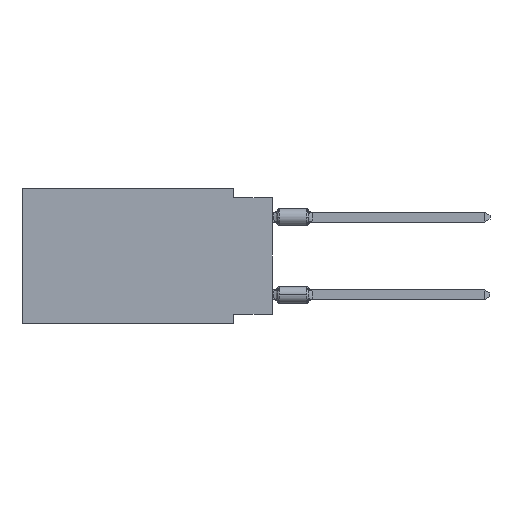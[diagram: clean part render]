
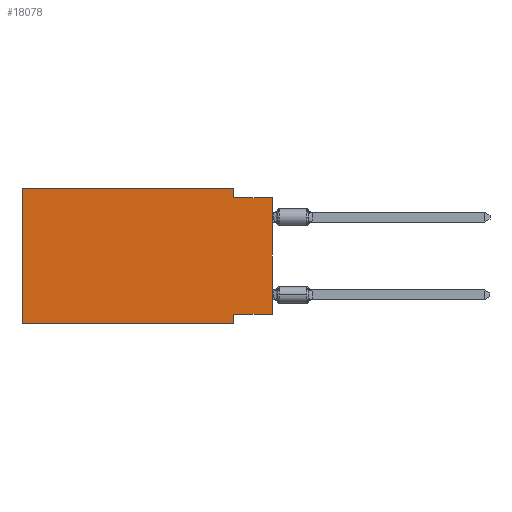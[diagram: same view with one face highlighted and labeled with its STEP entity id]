
A CAD part, left-side view. The second image highlights one B-rep face of the part: STEP entity #18078.
In plain terms, the highlighted planar face has unit normal (-1, 0, 0).
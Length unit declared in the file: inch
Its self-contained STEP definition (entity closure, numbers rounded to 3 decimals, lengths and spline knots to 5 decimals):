
#217 = VECTOR ( 'NONE', #5958, 39.37008 ) ;
#378 = EDGE_CURVE ( 'NONE', #1676, #13019, #11551, .T. ) ;
#433 = ORIENTED_EDGE ( 'NONE', *, *, #378, .F. ) ;
#554 = VERTEX_POINT ( 'NONE', #3143 ) ;
#1120 = CARTESIAN_POINT ( 'NONE',  ( 0., 0.645, 0. ) ) ;
#1152 = CARTESIAN_POINT ( 'NONE',  ( 0., 0.645, -0.35 ) ) ;
#1399 = CARTESIAN_POINT ( 'NONE',  ( 0., 0.645, 0. ) ) ;
#1676 = VERTEX_POINT ( 'NONE', #17907 ) ;
#1749 = CARTESIAN_POINT ( 'NONE',  ( 0., 0.645, 0. ) ) ;
#2171 = EDGE_CURVE ( 'NONE', #554, #13019, #19338, .T. ) ;
#2855 = EDGE_CURVE ( 'NONE', #4629, #8773, #21249, .T. ) ;
#3140 = CARTESIAN_POINT ( 'NONE',  ( 0., 0.1, 0. ) ) ;
#3143 = CARTESIAN_POINT ( 'NONE',  ( 0., 0.645, -0.35 ) ) ;
#3394 = VERTEX_POINT ( 'NONE', #15090 ) ;
#3724 = CARTESIAN_POINT ( 'NONE',  ( 0., 0., -0.025 ) ) ;
#4074 = LINE ( 'NONE', #7829, #217 ) ;
#4629 = VERTEX_POINT ( 'NONE', #1399 ) ;
#4888 = DIRECTION ( 'NONE',  ( 0., 0., -1. ) ) ;
#5103 = EDGE_CURVE ( 'NONE', #8773, #9860, #20241, .T. ) ;
#5451 = VERTEX_POINT ( 'NONE', #12352 ) ;
#5646 = DIRECTION ( 'NONE',  ( 0., -1., 0. ) ) ;
#5958 = DIRECTION ( 'NONE',  ( 0., 1., 0. ) ) ;
#6228 = ORIENTED_EDGE ( 'NONE', *, *, #2171, .T. ) ;
#6464 = CARTESIAN_POINT ( 'NONE',  ( 0., 0.1, 0. ) ) ;
#7521 = LINE ( 'NONE', #15108, #16155 ) ;
#7683 = AXIS2_PLACEMENT_3D ( 'NONE', #1120, #16372, #4888 ) ;
#7770 = DIRECTION ( 'NONE',  ( 0., 0., 1. ) ) ;
#7829 = CARTESIAN_POINT ( 'NONE',  ( 0., 0., -0.325 ) ) ;
#8244 = ORIENTED_EDGE ( 'NONE', *, *, #2855, .F. ) ;
#8361 = VECTOR ( 'NONE', #5646, 39.37008 ) ;
#8773 = VERTEX_POINT ( 'NONE', #6464 ) ;
#9860 = VERTEX_POINT ( 'NONE', #11965 ) ;
#10002 = VECTOR ( 'NONE', #13526, 39.37008 ) ;
#10067 = DIRECTION ( 'NONE',  ( 0., -1., 0. ) ) ;
#11280 = ORIENTED_EDGE ( 'NONE', *, *, #24445, .F. ) ;
#11551 = LINE ( 'NONE', #14797, #14588 ) ;
#11965 = CARTESIAN_POINT ( 'NONE',  ( 0., 0.1, -0.025 ) ) ;
#12352 = CARTESIAN_POINT ( 'NONE',  ( 0., 0., -0.025 ) ) ;
#12700 = EDGE_CURVE ( 'NONE', #3394, #1676, #4074, .T. ) ;
#13008 = ORIENTED_EDGE ( 'NONE', *, *, #21379, .F. ) ;
#13019 = VERTEX_POINT ( 'NONE', #20728 ) ;
#13526 = DIRECTION ( 'NONE',  ( 0., 0., 1. ) ) ;
#14370 = FACE_OUTER_BOUND ( 'NONE', #24104, .T. ) ;
#14588 = VECTOR ( 'NONE', #24274, 39.37008 ) ;
#14797 = CARTESIAN_POINT ( 'NONE',  ( 0., 0.1, -0.35 ) ) ;
#15090 = CARTESIAN_POINT ( 'NONE',  ( 0., 0., -0.325 ) ) ;
#15108 = CARTESIAN_POINT ( 'NONE',  ( 0., 0., 0. ) ) ;
#15766 = LINE ( 'NONE', #23378, #10002 ) ;
#16155 = VECTOR ( 'NONE', #7770, 39.37008 ) ;
#16372 = DIRECTION ( 'NONE',  ( 1., 0., 0. ) ) ;
#17907 = CARTESIAN_POINT ( 'NONE',  ( 0., 0.1, -0.325 ) ) ;
#18078 = ADVANCED_FACE ( 'NONE', ( #14370 ), #21970, .F. ) ;
#18663 = ORIENTED_EDGE ( 'NONE', *, *, #12700, .F. ) ;
#19338 = LINE ( 'NONE', #1152, #19974 ) ;
#19411 = ORIENTED_EDGE ( 'NONE', *, *, #5103, .F. ) ;
#19532 = VECTOR ( 'NONE', #10067, 39.37008 ) ;
#19785 = DIRECTION ( 'NONE',  ( 0., -1., 0. ) ) ;
#19974 = VECTOR ( 'NONE', #19785, 39.37008 ) ;
#20241 = LINE ( 'NONE', #3140, #22632 ) ;
#20728 = CARTESIAN_POINT ( 'NONE',  ( 0., 0.1, -0.35 ) ) ;
#20811 = LINE ( 'NONE', #3724, #19532 ) ;
#20833 = EDGE_CURVE ( 'NONE', #3394, #5451, #7521, .T. ) ;
#21249 = LINE ( 'NONE', #1749, #8361 ) ;
#21379 = EDGE_CURVE ( 'NONE', #9860, #5451, #20811, .T. ) ;
#21952 = ORIENTED_EDGE ( 'NONE', *, *, #20833, .T. ) ;
#21970 = PLANE ( 'NONE',  #7683 ) ;
#22344 = DIRECTION ( 'NONE',  ( 0., 0., -1. ) ) ;
#22632 = VECTOR ( 'NONE', #22344, 39.37008 ) ;
#23378 = CARTESIAN_POINT ( 'NONE',  ( 0., 0.645, 0. ) ) ;
#24104 = EDGE_LOOP ( 'NONE', ( #21952, #13008, #19411, #8244, #11280, #6228, #433, #18663 ) ) ;
#24274 = DIRECTION ( 'NONE',  ( 0., 0., -1. ) ) ;
#24445 = EDGE_CURVE ( 'NONE', #554, #4629, #15766, .T. ) ;
